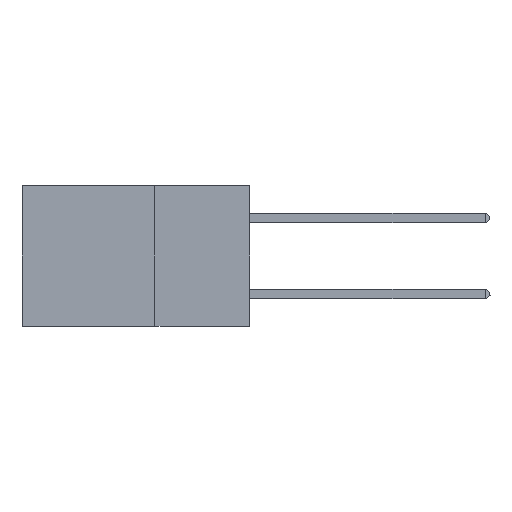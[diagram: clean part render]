
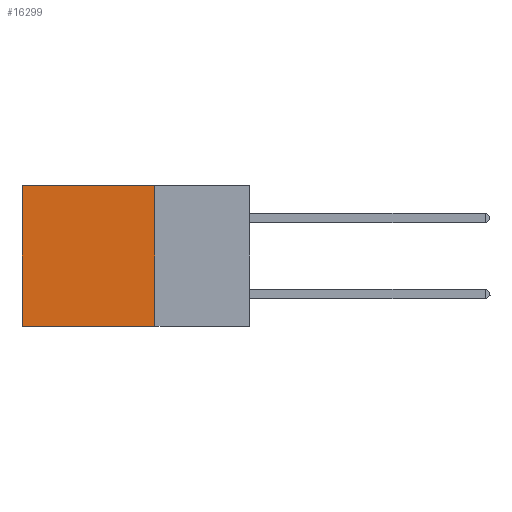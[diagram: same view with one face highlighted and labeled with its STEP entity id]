
A CAD part, left-side view. The second image highlights one B-rep face of the part: STEP entity #16299.
In plain terms, the highlighted planar face has unit normal (-1, 0, 0).
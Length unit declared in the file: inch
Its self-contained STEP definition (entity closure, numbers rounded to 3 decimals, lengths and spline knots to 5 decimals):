
#289 = CARTESIAN_POINT ( 'NONE',  ( 0.2875, 0.25, 0. ) ) ;
#611 = ORIENTED_EDGE ( 'NONE', *, *, #5581, .F. ) ;
#658 = LINE ( 'NONE', #11421, #9015 ) ;
#819 = VECTOR ( 'NONE', #14943, 39.37008 ) ;
#2061 = VERTEX_POINT ( 'NONE', #8560 ) ;
#3492 = ORIENTED_EDGE ( 'NONE', *, *, #14601, .F. ) ;
#3686 = EDGE_CURVE ( 'NONE', #13436, #2061, #658, .T. ) ;
#5340 = DIRECTION ( 'NONE',  ( 0., 1., 0. ) ) ;
#5342 = ORIENTED_EDGE ( 'NONE', *, *, #19764, .T. ) ;
#5364 = DIRECTION ( 'NONE',  ( 0., 0., -1. ) ) ;
#5581 = EDGE_CURVE ( 'NONE', #8811, #8962, #11152, .T. ) ;
#7577 = DIRECTION ( 'NONE',  ( 0., 0., -1. ) ) ;
#7606 = CARTESIAN_POINT ( 'NONE',  ( 0.2875, 0.25, 0. ) ) ;
#7659 = FACE_OUTER_BOUND ( 'NONE', #11513, .T. ) ;
#8560 = CARTESIAN_POINT ( 'NONE',  ( 0.2875, 0.6, -0.37 ) ) ;
#8811 = VERTEX_POINT ( 'NONE', #289 ) ;
#8962 = VERTEX_POINT ( 'NONE', #15960 ) ;
#9015 = VECTOR ( 'NONE', #5364, 39.37008 ) ;
#11028 = PLANE ( 'NONE',  #12844 ) ;
#11152 = LINE ( 'NONE', #11873, #14912 ) ;
#11421 = CARTESIAN_POINT ( 'NONE',  ( 0.2875, 0.6, 0. ) ) ;
#11513 = EDGE_LOOP ( 'NONE', ( #17243, #3492, #611, #5342 ) ) ;
#11873 = CARTESIAN_POINT ( 'NONE',  ( 0.2875, 0.25, 0. ) ) ;
#12548 = CARTESIAN_POINT ( 'NONE',  ( 0.2875, 0.25, 0. ) ) ;
#12844 = AXIS2_PLACEMENT_3D ( 'NONE', #12548, #15571, #7577 ) ;
#12892 = CARTESIAN_POINT ( 'NONE',  ( 0.2875, 0.6, 0. ) ) ;
#13436 = VERTEX_POINT ( 'NONE', #12892 ) ;
#13569 = CARTESIAN_POINT ( 'NONE',  ( 0.2875, 0.25, -0.37 ) ) ;
#13695 = LINE ( 'NONE', #13569, #17421 ) ;
#14601 = EDGE_CURVE ( 'NONE', #8962, #2061, #13695, .T. ) ;
#14912 = VECTOR ( 'NONE', #18441, 39.37008 ) ;
#14943 = DIRECTION ( 'NONE',  ( 0., 1., 0. ) ) ;
#15571 = DIRECTION ( 'NONE',  ( 1., 0., 0. ) ) ;
#15960 = CARTESIAN_POINT ( 'NONE',  ( 0.2875, 0.25, -0.37 ) ) ;
#16299 = ADVANCED_FACE ( 'NONE', ( #7659 ), #11028, .F. ) ;
#17243 = ORIENTED_EDGE ( 'NONE', *, *, #3686, .T. ) ;
#17421 = VECTOR ( 'NONE', #5340, 39.37008 ) ;
#17888 = LINE ( 'NONE', #7606, #819 ) ;
#18441 = DIRECTION ( 'NONE',  ( 0., 0., -1. ) ) ;
#19764 = EDGE_CURVE ( 'NONE', #8811, #13436, #17888, .T. ) ;
